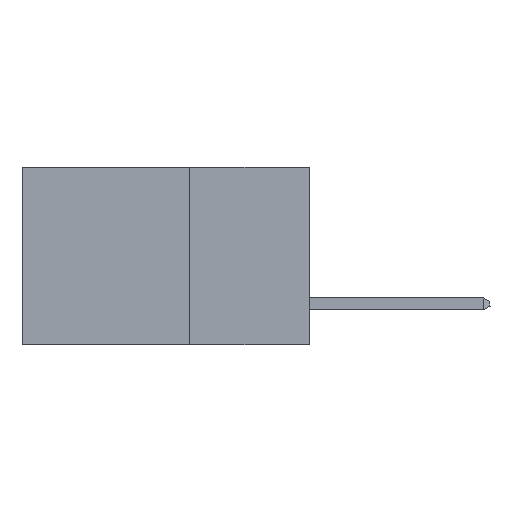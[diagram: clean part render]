
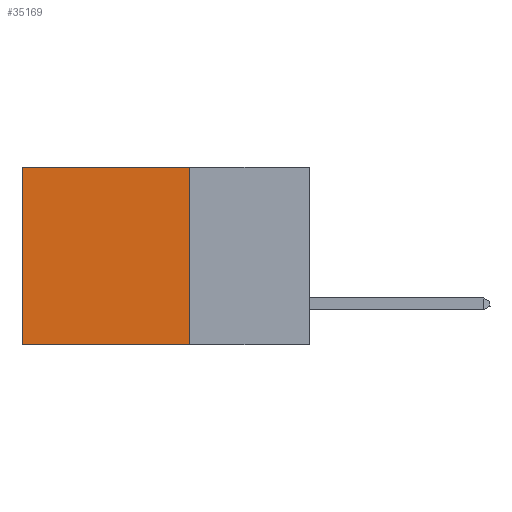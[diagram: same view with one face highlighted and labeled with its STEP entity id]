
A CAD part, left-side view. The second image highlights one B-rep face of the part: STEP entity #35169.
In plain terms, the highlighted planar face has unit normal (-1, 0, 0).
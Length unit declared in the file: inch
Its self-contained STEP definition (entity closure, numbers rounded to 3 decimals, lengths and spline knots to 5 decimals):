
#720 = CARTESIAN_POINT ( 'NONE',  ( 0.2875, 0.25, -0.37 ) ) ;
#1420 = CARTESIAN_POINT ( 'NONE',  ( 0.2875, 0.25, 0. ) ) ;
#2266 = CARTESIAN_POINT ( 'NONE',  ( 0.2875, 0.25, 0. ) ) ;
#2443 = DIRECTION ( 'NONE',  ( 0., 0., -1. ) ) ;
#2856 = VECTOR ( 'NONE', #48930, 39.37008 ) ;
#4093 = LINE ( 'NONE', #17378, #2856 ) ;
#4735 = VECTOR ( 'NONE', #43662, 39.37008 ) ;
#6135 = EDGE_CURVE ( 'NONE', #24520, #22320, #4093, .T. ) ;
#6165 = VERTEX_POINT ( 'NONE', #24969 ) ;
#8220 = EDGE_LOOP ( 'NONE', ( #11833, #14919, #23802, #48330 ) ) ;
#11833 = ORIENTED_EDGE ( 'NONE', *, *, #38469, .T. ) ;
#12154 = VERTEX_POINT ( 'NONE', #41649 ) ;
#12469 = LINE ( 'NONE', #720, #26034 ) ;
#12740 = VECTOR ( 'NONE', #41207, 39.37008 ) ;
#12944 = CARTESIAN_POINT ( 'NONE',  ( 0.2875, 0.25, 0. ) ) ;
#14234 = EDGE_CURVE ( 'NONE', #24520, #6165, #36830, .T. ) ;
#14919 = ORIENTED_EDGE ( 'NONE', *, *, #25418, .F. ) ;
#15950 = CARTESIAN_POINT ( 'NONE',  ( 0.2875, 0.6, 0. ) ) ;
#17378 = CARTESIAN_POINT ( 'NONE',  ( 0.2875, 0.25, 0. ) ) ;
#22141 = DIRECTION ( 'NONE',  ( 1., 0., 0. ) ) ;
#22320 = VERTEX_POINT ( 'NONE', #22967 ) ;
#22967 = CARTESIAN_POINT ( 'NONE',  ( 0.2875, 0.25, -0.37 ) ) ;
#23802 = ORIENTED_EDGE ( 'NONE', *, *, #6135, .F. ) ;
#24520 = VERTEX_POINT ( 'NONE', #12944 ) ;
#24969 = CARTESIAN_POINT ( 'NONE',  ( 0.2875, 0.6, 0. ) ) ;
#25418 = EDGE_CURVE ( 'NONE', #22320, #12154, #12469, .T. ) ;
#26034 = VECTOR ( 'NONE', #37813, 39.37008 ) ;
#26087 = PLANE ( 'NONE',  #38064 ) ;
#28853 = LINE ( 'NONE', #15950, #4735 ) ;
#35169 = ADVANCED_FACE ( 'NONE', ( #36418 ), #26087, .F. ) ;
#36418 = FACE_OUTER_BOUND ( 'NONE', #8220, .T. ) ;
#36830 = LINE ( 'NONE', #1420, #12740 ) ;
#37813 = DIRECTION ( 'NONE',  ( 0., 1., 0. ) ) ;
#38064 = AXIS2_PLACEMENT_3D ( 'NONE', #2266, #22141, #2443 ) ;
#38469 = EDGE_CURVE ( 'NONE', #6165, #12154, #28853, .T. ) ;
#41207 = DIRECTION ( 'NONE',  ( 0., 1., 0. ) ) ;
#41649 = CARTESIAN_POINT ( 'NONE',  ( 0.2875, 0.6, -0.37 ) ) ;
#43662 = DIRECTION ( 'NONE',  ( 0., 0., -1. ) ) ;
#48330 = ORIENTED_EDGE ( 'NONE', *, *, #14234, .T. ) ;
#48930 = DIRECTION ( 'NONE',  ( 0., 0., -1. ) ) ;
